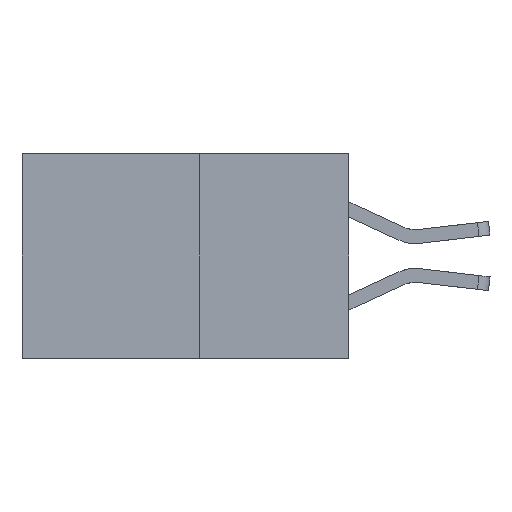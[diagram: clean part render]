
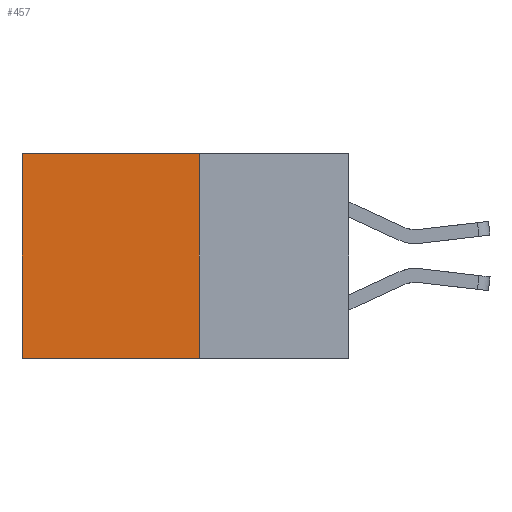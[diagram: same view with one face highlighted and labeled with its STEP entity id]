
A CAD part, left-side view. The second image highlights one B-rep face of the part: STEP entity #457.
In plain terms, the highlighted planar face has unit normal (-1, 0, 0).
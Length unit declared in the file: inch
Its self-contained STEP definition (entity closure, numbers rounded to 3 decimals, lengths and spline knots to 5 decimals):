
#457 = ADVANCED_FACE ( 'NONE', ( #7300 ), #2393, .F. ) ;
#516 = CARTESIAN_POINT ( 'NONE',  ( 0.277, 0.27, -0.37 ) ) ;
#996 = ORIENTED_EDGE ( 'NONE', *, *, #7576, .T. ) ;
#1140 = DIRECTION ( 'NONE',  ( 0., 0., -1. ) ) ;
#1205 = ORIENTED_EDGE ( 'NONE', *, *, #1503, .F. ) ;
#1246 = DIRECTION ( 'NONE',  ( 0., 1., 0. ) ) ;
#1462 = CARTESIAN_POINT ( 'NONE',  ( 0.277, 0.27, -0.37 ) ) ;
#1503 = EDGE_CURVE ( 'NONE', #5024, #10576, #6671, .T. ) ;
#1602 = EDGE_CURVE ( 'NONE', #2828, #10576, #1618, .T. ) ;
#1618 = LINE ( 'NONE', #3942, #3925 ) ;
#1849 = CARTESIAN_POINT ( 'NONE',  ( 0.277, 0.27, -0.37 ) ) ;
#1852 = DIRECTION ( 'NONE',  ( 0., 1., 0. ) ) ;
#1929 = AXIS2_PLACEMENT_3D ( 'NONE', #1849, #6790, #5234 ) ;
#1987 = CARTESIAN_POINT ( 'NONE',  ( 0.277, 0.27, -0.37 ) ) ;
#2152 = VECTOR ( 'NONE', #1852, 39.37008 ) ;
#2393 = PLANE ( 'NONE',  #1929 ) ;
#2828 = VERTEX_POINT ( 'NONE', #8999 ) ;
#3925 = VECTOR ( 'NONE', #1140, 39.37008 ) ;
#3942 = CARTESIAN_POINT ( 'NONE',  ( 0.277, 0.59, -0.37 ) ) ;
#5024 = VERTEX_POINT ( 'NONE', #1987 ) ;
#5114 = EDGE_LOOP ( 'NONE', ( #7913, #1205, #8353, #996 ) ) ;
#5234 = DIRECTION ( 'NONE',  ( 0., 0., -1. ) ) ;
#5237 = CARTESIAN_POINT ( 'NONE',  ( 0.277, 0.27, 0. ) ) ;
#5501 = CARTESIAN_POINT ( 'NONE',  ( 0.277, 0.27, 0. ) ) ;
#5550 = VECTOR ( 'NONE', #8885, 39.37008 ) ;
#6196 = EDGE_CURVE ( 'NONE', #10325, #5024, #7719, .T. ) ;
#6671 = LINE ( 'NONE', #1462, #2152 ) ;
#6790 = DIRECTION ( 'NONE',  ( 1., 0., 0. ) ) ;
#7300 = FACE_OUTER_BOUND ( 'NONE', #5114, .T. ) ;
#7576 = EDGE_CURVE ( 'NONE', #10325, #2828, #9594, .T. ) ;
#7719 = LINE ( 'NONE', #516, #5550 ) ;
#7913 = ORIENTED_EDGE ( 'NONE', *, *, #1602, .T. ) ;
#7941 = VECTOR ( 'NONE', #1246, 39.37008 ) ;
#8353 = ORIENTED_EDGE ( 'NONE', *, *, #6196, .F. ) ;
#8885 = DIRECTION ( 'NONE',  ( 0., 0., -1. ) ) ;
#8999 = CARTESIAN_POINT ( 'NONE',  ( 0.277, 0.59, 0. ) ) ;
#9594 = LINE ( 'NONE', #5501, #7941 ) ;
#9679 = CARTESIAN_POINT ( 'NONE',  ( 0.277, 0.59, -0.37 ) ) ;
#10325 = VERTEX_POINT ( 'NONE', #5237 ) ;
#10576 = VERTEX_POINT ( 'NONE', #9679 ) ;
